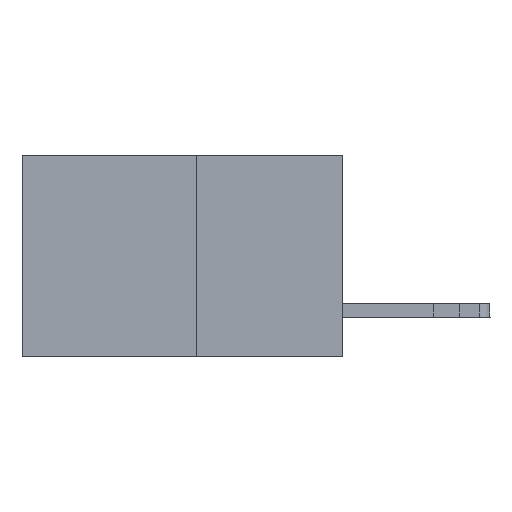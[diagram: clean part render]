
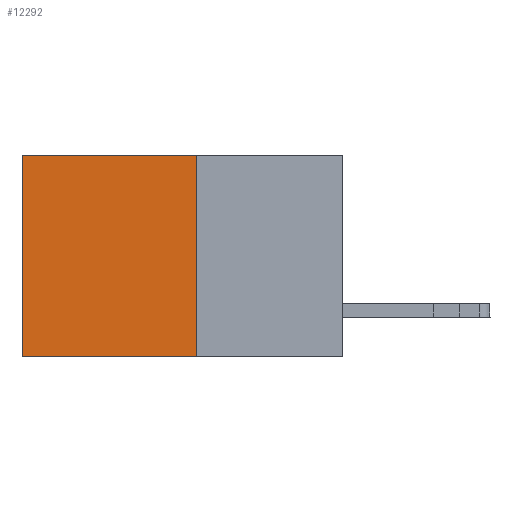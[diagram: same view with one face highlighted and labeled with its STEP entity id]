
A CAD part, left-side view. The second image highlights one B-rep face of the part: STEP entity #12292.
In plain terms, the highlighted planar face has unit normal (-1, 0, 0).
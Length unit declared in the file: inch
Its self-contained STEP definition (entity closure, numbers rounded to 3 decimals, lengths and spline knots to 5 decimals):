
#412 = EDGE_CURVE ( 'NONE', #16419, #3819, #5861, .T. ) ;
#657 = CARTESIAN_POINT ( 'NONE',  ( 0.277, 0.27, -0.37 ) ) ;
#2820 = CARTESIAN_POINT ( 'NONE',  ( 0.277, 0.27, -0.37 ) ) ;
#3550 = CARTESIAN_POINT ( 'NONE',  ( 0.277, 0.27, 0. ) ) ;
#3679 = LINE ( 'NONE', #657, #5310 ) ;
#3819 = VERTEX_POINT ( 'NONE', #5537 ) ;
#3851 = DIRECTION ( 'NONE',  ( 0., 0., -1. ) ) ;
#5060 = VERTEX_POINT ( 'NONE', #3550 ) ;
#5172 = VECTOR ( 'NONE', #10090, 39.37008 ) ;
#5232 = AXIS2_PLACEMENT_3D ( 'NONE', #2820, #7036, #14974 ) ;
#5310 = VECTOR ( 'NONE', #13976, 39.37008 ) ;
#5482 = VERTEX_POINT ( 'NONE', #10055 ) ;
#5529 = PLANE ( 'NONE',  #5232 ) ;
#5537 = CARTESIAN_POINT ( 'NONE',  ( 0.277, 0.59, -0.37 ) ) ;
#5861 = LINE ( 'NONE', #16869, #5172 ) ;
#5961 = EDGE_LOOP ( 'NONE', ( #11571, #7078, #10566, #13191 ) ) ;
#7036 = DIRECTION ( 'NONE',  ( 1., 0., 0. ) ) ;
#7078 = ORIENTED_EDGE ( 'NONE', *, *, #10907, .F. ) ;
#9587 = FACE_OUTER_BOUND ( 'NONE', #5961, .T. ) ;
#10055 = CARTESIAN_POINT ( 'NONE',  ( 0.277, 0.27, -0.37 ) ) ;
#10090 = DIRECTION ( 'NONE',  ( 0., 0., -1. ) ) ;
#10566 = ORIENTED_EDGE ( 'NONE', *, *, #12644, .F. ) ;
#10907 = EDGE_CURVE ( 'NONE', #5482, #3819, #3679, .T. ) ;
#11571 = ORIENTED_EDGE ( 'NONE', *, *, #412, .T. ) ;
#11770 = LINE ( 'NONE', #15831, #11951 ) ;
#11951 = VECTOR ( 'NONE', #3851, 39.37008 ) ;
#12292 = ADVANCED_FACE ( 'NONE', ( #9587 ), #5529, .F. ) ;
#12644 = EDGE_CURVE ( 'NONE', #5060, #5482, #11770, .T. ) ;
#13191 = ORIENTED_EDGE ( 'NONE', *, *, #16914, .T. ) ;
#13976 = DIRECTION ( 'NONE',  ( 0., 1., 0. ) ) ;
#14796 = VECTOR ( 'NONE', #16488, 39.37008 ) ;
#14974 = DIRECTION ( 'NONE',  ( 0., 0., -1. ) ) ;
#15176 = CARTESIAN_POINT ( 'NONE',  ( 0.277, 0.27, 0. ) ) ;
#15831 = CARTESIAN_POINT ( 'NONE',  ( 0.277, 0.27, -0.37 ) ) ;
#16419 = VERTEX_POINT ( 'NONE', #16678 ) ;
#16488 = DIRECTION ( 'NONE',  ( 0., 1., 0. ) ) ;
#16569 = LINE ( 'NONE', #15176, #14796 ) ;
#16678 = CARTESIAN_POINT ( 'NONE',  ( 0.277, 0.59, 0. ) ) ;
#16869 = CARTESIAN_POINT ( 'NONE',  ( 0.277, 0.59, -0.37 ) ) ;
#16914 = EDGE_CURVE ( 'NONE', #5060, #16419, #16569, .T. ) ;
